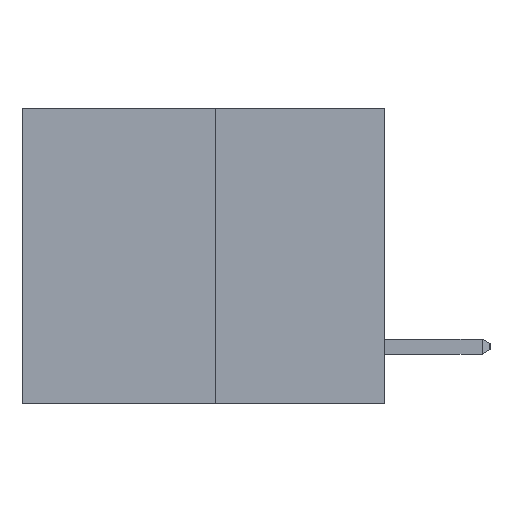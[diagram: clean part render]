
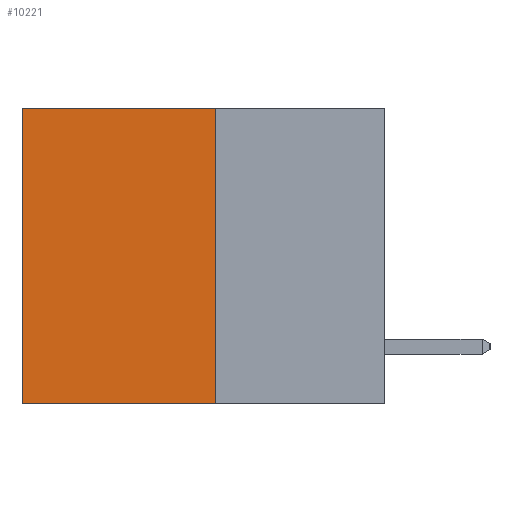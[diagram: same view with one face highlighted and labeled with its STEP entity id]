
A CAD part, left-side view. The second image highlights one B-rep face of the part: STEP entity #10221.
In plain terms, the highlighted planar face has unit normal (-1, 0, 0).
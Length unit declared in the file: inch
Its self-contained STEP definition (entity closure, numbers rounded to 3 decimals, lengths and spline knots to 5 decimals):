
#176 = ORIENTED_EDGE ( 'NONE', *, *, #8528, .F. ) ;
#869 = CARTESIAN_POINT ( 'NONE',  ( 0.3165, 0.28, -0.49 ) ) ;
#2286 = VERTEX_POINT ( 'NONE', #4362 ) ;
#2477 = LINE ( 'NONE', #9255, #10313 ) ;
#3267 = DIRECTION ( 'NONE',  ( 0., 1., 0. ) ) ;
#4362 = CARTESIAN_POINT ( 'NONE',  ( 0.3165, 0.6, -0.49 ) ) ;
#4522 = EDGE_LOOP ( 'NONE', ( #5254, #176, #12501, #6300 ) ) ;
#4639 = PLANE ( 'NONE',  #8577 ) ;
#4933 = DIRECTION ( 'NONE',  ( 0., 0., -1. ) ) ;
#5104 = CARTESIAN_POINT ( 'NONE',  ( 0.3165, 0.6, -0.49 ) ) ;
#5254 = ORIENTED_EDGE ( 'NONE', *, *, #15760, .T. ) ;
#5746 = LINE ( 'NONE', #14080, #8517 ) ;
#5763 = EDGE_CURVE ( 'NONE', #8635, #12374, #2477, .T. ) ;
#6099 = FACE_OUTER_BOUND ( 'NONE', #4522, .T. ) ;
#6191 = DIRECTION ( 'NONE',  ( 0., 0., -1. ) ) ;
#6300 = ORIENTED_EDGE ( 'NONE', *, *, #5763, .T. ) ;
#7082 = EDGE_CURVE ( 'NONE', #8635, #17373, #15545, .T. ) ;
#7212 = CARTESIAN_POINT ( 'NONE',  ( 0.3165, 0.28, 0. ) ) ;
#7355 = DIRECTION ( 'NONE',  ( 1., 0., 0. ) ) ;
#7729 = VECTOR ( 'NONE', #9584, 39.37008 ) ;
#8517 = VECTOR ( 'NONE', #3267, 39.37008 ) ;
#8528 = EDGE_CURVE ( 'NONE', #17373, #2286, #5746, .T. ) ;
#8577 = AXIS2_PLACEMENT_3D ( 'NONE', #16872, #7355, #4933 ) ;
#8635 = VERTEX_POINT ( 'NONE', #7212 ) ;
#9255 = CARTESIAN_POINT ( 'NONE',  ( 0.3165, 0.28, 0. ) ) ;
#9584 = DIRECTION ( 'NONE',  ( 0., 0., -1. ) ) ;
#10221 = ADVANCED_FACE ( 'NONE', ( #6099 ), #4639, .F. ) ;
#10243 = CARTESIAN_POINT ( 'NONE',  ( 0.3165, 0.28, -0.49 ) ) ;
#10313 = VECTOR ( 'NONE', #11964, 39.37008 ) ;
#11832 = LINE ( 'NONE', #5104, #17094 ) ;
#11964 = DIRECTION ( 'NONE',  ( 0., 1., 0. ) ) ;
#12374 = VERTEX_POINT ( 'NONE', #17410 ) ;
#12501 = ORIENTED_EDGE ( 'NONE', *, *, #7082, .F. ) ;
#14080 = CARTESIAN_POINT ( 'NONE',  ( 0.3165, 0.28, -0.49 ) ) ;
#15545 = LINE ( 'NONE', #10243, #7729 ) ;
#15760 = EDGE_CURVE ( 'NONE', #12374, #2286, #11832, .T. ) ;
#16872 = CARTESIAN_POINT ( 'NONE',  ( 0.3165, 0.28, -0.49 ) ) ;
#17094 = VECTOR ( 'NONE', #6191, 39.37008 ) ;
#17373 = VERTEX_POINT ( 'NONE', #869 ) ;
#17410 = CARTESIAN_POINT ( 'NONE',  ( 0.3165, 0.6, 0. ) ) ;
